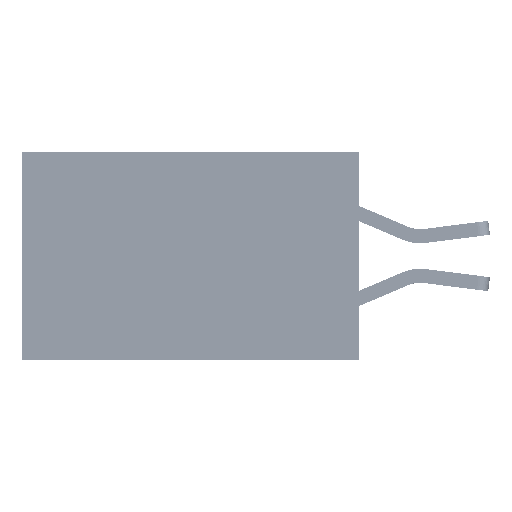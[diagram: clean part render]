
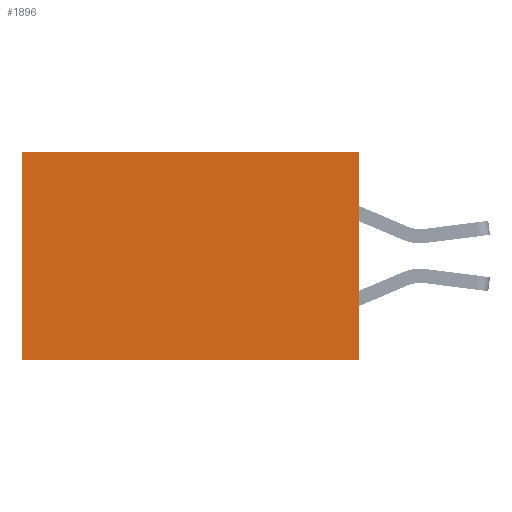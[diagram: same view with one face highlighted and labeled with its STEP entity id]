
A CAD part, left-side view. The second image highlights one B-rep face of the part: STEP entity #1896.
In plain terms, the highlighted planar face has unit normal (-1, 0, 0).
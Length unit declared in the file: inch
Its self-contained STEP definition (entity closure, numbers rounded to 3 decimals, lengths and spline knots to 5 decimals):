
#452 = CARTESIAN_POINT ( 'NONE',  ( 0.2875, 0., -0.37 ) ) ;
#1070 = EDGE_CURVE ( 'NONE', #22425, #24318, #29496, .T. ) ;
#1094 = EDGE_CURVE ( 'NONE', #24318, #13181, #36041, .T. ) ;
#1510 = CARTESIAN_POINT ( 'NONE',  ( 0.2875, 0., 0. ) ) ;
#1896 = ADVANCED_FACE ( 'NONE', ( #22729 ), #35697, .F. ) ;
#3264 = DIRECTION ( 'NONE',  ( 0., 1., 0. ) ) ;
#4718 = VERTEX_POINT ( 'NONE', #25675 ) ;
#6565 = AXIS2_PLACEMENT_3D ( 'NONE', #1510, #30077, #37376 ) ;
#6707 = CARTESIAN_POINT ( 'NONE',  ( 0.2875, 0., 0. ) ) ;
#7673 = ORIENTED_EDGE ( 'NONE', *, *, #14607, .T. ) ;
#8870 = DIRECTION ( 'NONE',  ( 0., 0., -1. ) ) ;
#9079 = DIRECTION ( 'NONE',  ( 0., 1., 0. ) ) ;
#10326 = CARTESIAN_POINT ( 'NONE',  ( 0.2875, 0.6, -0.37 ) ) ;
#10470 = LINE ( 'NONE', #28665, #19636 ) ;
#10528 = LINE ( 'NONE', #31697, #35512 ) ;
#11215 = EDGE_CURVE ( 'NONE', #22425, #4718, #10470, .T. ) ;
#13181 = VERTEX_POINT ( 'NONE', #10326 ) ;
#14607 = EDGE_CURVE ( 'NONE', #4718, #13181, #10528, .T. ) ;
#14864 = ORIENTED_EDGE ( 'NONE', *, *, #1070, .F. ) ;
#16541 = ORIENTED_EDGE ( 'NONE', *, *, #1094, .F. ) ;
#18779 = VECTOR ( 'NONE', #3264, 39.37008 ) ;
#19636 = VECTOR ( 'NONE', #9079, 39.37008 ) ;
#19723 = CARTESIAN_POINT ( 'NONE',  ( 0.2875, 0., -0.37 ) ) ;
#20585 = CARTESIAN_POINT ( 'NONE',  ( 0.2875, 0., 0. ) ) ;
#20810 = VECTOR ( 'NONE', #26264, 39.37008 ) ;
#22425 = VERTEX_POINT ( 'NONE', #20585 ) ;
#22729 = FACE_OUTER_BOUND ( 'NONE', #34317, .T. ) ;
#24318 = VERTEX_POINT ( 'NONE', #452 ) ;
#25675 = CARTESIAN_POINT ( 'NONE',  ( 0.2875, 0.6, 0. ) ) ;
#26264 = DIRECTION ( 'NONE',  ( 0., 0., -1. ) ) ;
#28665 = CARTESIAN_POINT ( 'NONE',  ( 0.2875, 0., 0. ) ) ;
#29496 = LINE ( 'NONE', #6707, #20810 ) ;
#30077 = DIRECTION ( 'NONE',  ( 1., 0., 0. ) ) ;
#31697 = CARTESIAN_POINT ( 'NONE',  ( 0.2875, 0.6, 0. ) ) ;
#34317 = EDGE_LOOP ( 'NONE', ( #7673, #16541, #14864, #41420 ) ) ;
#35512 = VECTOR ( 'NONE', #8870, 39.37008 ) ;
#35697 = PLANE ( 'NONE',  #6565 ) ;
#36041 = LINE ( 'NONE', #19723, #18779 ) ;
#37376 = DIRECTION ( 'NONE',  ( 0., 0., -1. ) ) ;
#41420 = ORIENTED_EDGE ( 'NONE', *, *, #11215, .T. ) ;
